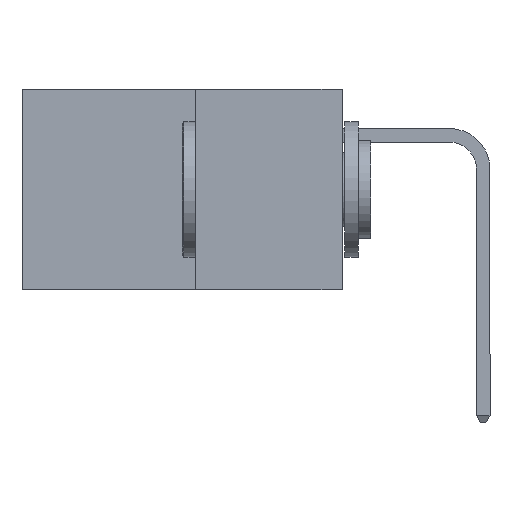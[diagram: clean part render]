
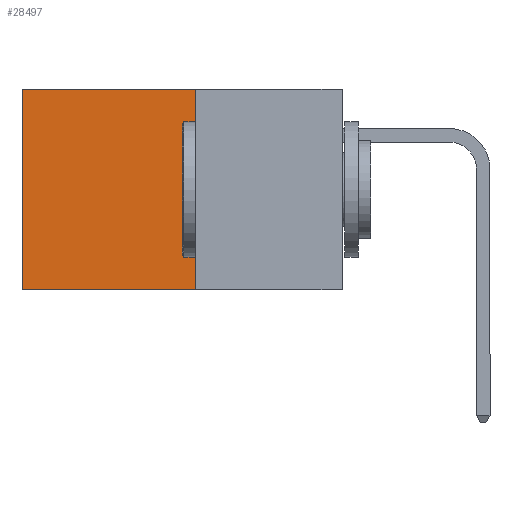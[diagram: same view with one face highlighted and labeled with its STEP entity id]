
A CAD part, left-side view. The second image highlights one B-rep face of the part: STEP entity #28497.
In plain terms, the highlighted planar face has unit normal (-1, 0, 0).
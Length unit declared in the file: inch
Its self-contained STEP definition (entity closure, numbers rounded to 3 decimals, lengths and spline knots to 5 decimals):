
#201 = ORIENTED_EDGE ( 'NONE', *, *, #9882, .F. ) ;
#244 = EDGE_CURVE ( 'NONE', #15805, #12357, #4870, .T. ) ;
#560 = VECTOR ( 'NONE', #14793, 39.37008 ) ;
#2425 = ORIENTED_EDGE ( 'NONE', *, *, #24829, .F. ) ;
#4870 = LINE ( 'NONE', #27801, #16890 ) ;
#6208 = PLANE ( 'NONE',  #13406 ) ;
#6210 = CARTESIAN_POINT ( 'NONE',  ( 0.277, 0.27, -0.37 ) ) ;
#6888 = CARTESIAN_POINT ( 'NONE',  ( 0.277, 0.59, 0. ) ) ;
#8493 = CARTESIAN_POINT ( 'NONE',  ( 0.277, 0.59, -0.37 ) ) ;
#8914 = FACE_OUTER_BOUND ( 'NONE', #9232, .T. ) ;
#9232 = EDGE_LOOP ( 'NONE', ( #23082, #201, #2425, #23718 ) ) ;
#9293 = VERTEX_POINT ( 'NONE', #18421 ) ;
#9536 = LINE ( 'NONE', #6210, #15940 ) ;
#9882 = EDGE_CURVE ( 'NONE', #21258, #12357, #9536, .T. ) ;
#11062 = DIRECTION ( 'NONE',  ( 1., 0., 0. ) ) ;
#12357 = VERTEX_POINT ( 'NONE', #8493 ) ;
#12362 = CARTESIAN_POINT ( 'NONE',  ( 0.277, 0.27, 0. ) ) ;
#13406 = AXIS2_PLACEMENT_3D ( 'NONE', #25454, #11062, #27851 ) ;
#14793 = DIRECTION ( 'NONE',  ( 0., 1., 0. ) ) ;
#15805 = VERTEX_POINT ( 'NONE', #6888 ) ;
#15940 = VECTOR ( 'NONE', #23029, 39.37008 ) ;
#16564 = VECTOR ( 'NONE', #22811, 39.37008 ) ;
#16890 = VECTOR ( 'NONE', #24174, 39.37008 ) ;
#16990 = CARTESIAN_POINT ( 'NONE',  ( 0.277, 0.27, -0.37 ) ) ;
#18421 = CARTESIAN_POINT ( 'NONE',  ( 0.277, 0.27, 0. ) ) ;
#19517 = EDGE_CURVE ( 'NONE', #9293, #15805, #19755, .T. ) ;
#19755 = LINE ( 'NONE', #12362, #560 ) ;
#20358 = CARTESIAN_POINT ( 'NONE',  ( 0.277, 0.27, -0.37 ) ) ;
#21258 = VERTEX_POINT ( 'NONE', #16990 ) ;
#22811 = DIRECTION ( 'NONE',  ( 0., 0., -1. ) ) ;
#23029 = DIRECTION ( 'NONE',  ( 0., 1., 0. ) ) ;
#23082 = ORIENTED_EDGE ( 'NONE', *, *, #244, .T. ) ;
#23718 = ORIENTED_EDGE ( 'NONE', *, *, #19517, .T. ) ;
#24174 = DIRECTION ( 'NONE',  ( 0., 0., -1. ) ) ;
#24829 = EDGE_CURVE ( 'NONE', #9293, #21258, #29290, .T. ) ;
#25454 = CARTESIAN_POINT ( 'NONE',  ( 0.277, 0.27, -0.37 ) ) ;
#27801 = CARTESIAN_POINT ( 'NONE',  ( 0.277, 0.59, -0.37 ) ) ;
#27851 = DIRECTION ( 'NONE',  ( 0., 0., -1. ) ) ;
#28497 = ADVANCED_FACE ( 'NONE', ( #8914 ), #6208, .F. ) ;
#29290 = LINE ( 'NONE', #20358, #16564 ) ;
